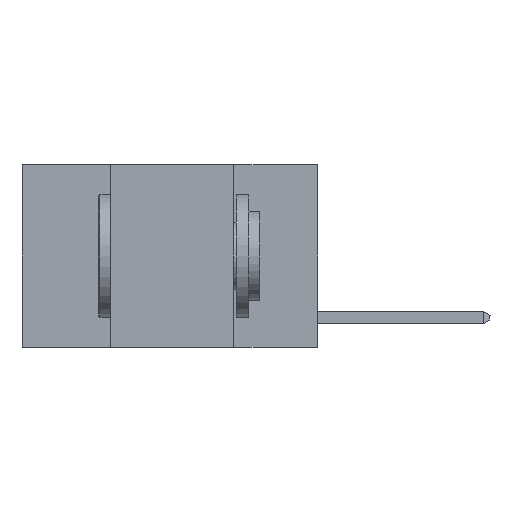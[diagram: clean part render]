
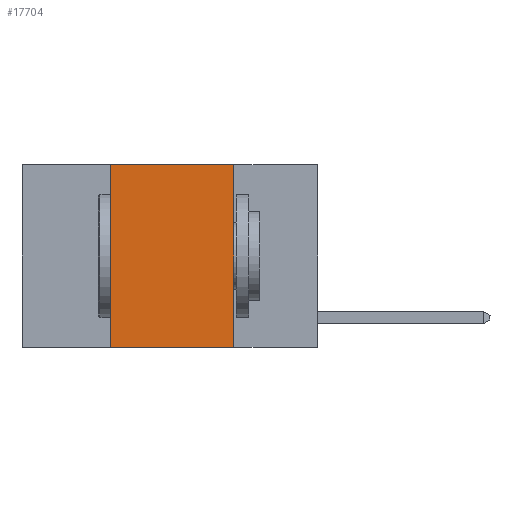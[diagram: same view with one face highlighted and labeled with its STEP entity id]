
A CAD part, left-side view. The second image highlights one B-rep face of the part: STEP entity #17704.
In plain terms, the highlighted planar face has unit normal (-1, 0, 0).
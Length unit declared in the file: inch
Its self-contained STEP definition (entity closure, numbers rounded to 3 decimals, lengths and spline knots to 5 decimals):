
#364 = CARTESIAN_POINT ( 'NONE',  ( 0., 0.42, -0.37 ) ) ;
#509 = LINE ( 'NONE', #11505, #6200 ) ;
#534 = ORIENTED_EDGE ( 'NONE', *, *, #3186, .F. ) ;
#2205 = DIRECTION ( 'NONE',  ( 1., 0., 0. ) ) ;
#2339 = VECTOR ( 'NONE', #5417, 39.37008 ) ;
#2409 = LINE ( 'NONE', #18168, #2339 ) ;
#2705 = CARTESIAN_POINT ( 'NONE',  ( 0., 0.17, 0. ) ) ;
#2998 = CARTESIAN_POINT ( 'NONE',  ( 0., 0.42, 0. ) ) ;
#3186 = EDGE_CURVE ( 'NONE', #4792, #4472, #509, .T. ) ;
#4249 = ORIENTED_EDGE ( 'NONE', *, *, #5875, .F. ) ;
#4472 = VERTEX_POINT ( 'NONE', #8131 ) ;
#4792 = VERTEX_POINT ( 'NONE', #2705 ) ;
#5259 = DIRECTION ( 'NONE',  ( 0., 0., 1. ) ) ;
#5417 = DIRECTION ( 'NONE',  ( 0., -1., 0. ) ) ;
#5708 = CARTESIAN_POINT ( 'NONE',  ( 0., 0.6, 0. ) ) ;
#5875 = EDGE_CURVE ( 'NONE', #7694, #4792, #2409, .T. ) ;
#6200 = VECTOR ( 'NONE', #19288, 39.37008 ) ;
#6436 = EDGE_LOOP ( 'NONE', ( #534, #4249, #13382, #18983 ) ) ;
#7178 = FACE_OUTER_BOUND ( 'NONE', #6436, .T. ) ;
#7283 = PLANE ( 'NONE',  #17291 ) ;
#7694 = VERTEX_POINT ( 'NONE', #2998 ) ;
#8131 = CARTESIAN_POINT ( 'NONE',  ( 0., 0.17, -0.37 ) ) ;
#8898 = LINE ( 'NONE', #12017, #10555 ) ;
#9876 = EDGE_CURVE ( 'NONE', #18454, #7694, #11695, .T. ) ;
#10555 = VECTOR ( 'NONE', #15202, 39.37008 ) ;
#10866 = VECTOR ( 'NONE', #5259, 39.37008 ) ;
#11505 = CARTESIAN_POINT ( 'NONE',  ( 0., 0.17, 0. ) ) ;
#11695 = LINE ( 'NONE', #19473, #10866 ) ;
#11942 = EDGE_CURVE ( 'NONE', #18454, #4472, #8898, .T. ) ;
#12017 = CARTESIAN_POINT ( 'NONE',  ( 0., 0.6, -0.37 ) ) ;
#13382 = ORIENTED_EDGE ( 'NONE', *, *, #9876, .F. ) ;
#15202 = DIRECTION ( 'NONE',  ( 0., -1., 0. ) ) ;
#17291 = AXIS2_PLACEMENT_3D ( 'NONE', #5708, #2205, #18061 ) ;
#17704 = ADVANCED_FACE ( 'NONE', ( #7178 ), #7283, .F. ) ;
#18061 = DIRECTION ( 'NONE',  ( 0., 0., -1. ) ) ;
#18168 = CARTESIAN_POINT ( 'NONE',  ( 0., 0.6, 0. ) ) ;
#18454 = VERTEX_POINT ( 'NONE', #364 ) ;
#18983 = ORIENTED_EDGE ( 'NONE', *, *, #11942, .T. ) ;
#19288 = DIRECTION ( 'NONE',  ( 0., 0., -1. ) ) ;
#19473 = CARTESIAN_POINT ( 'NONE',  ( 0., 0.42, 0. ) ) ;
